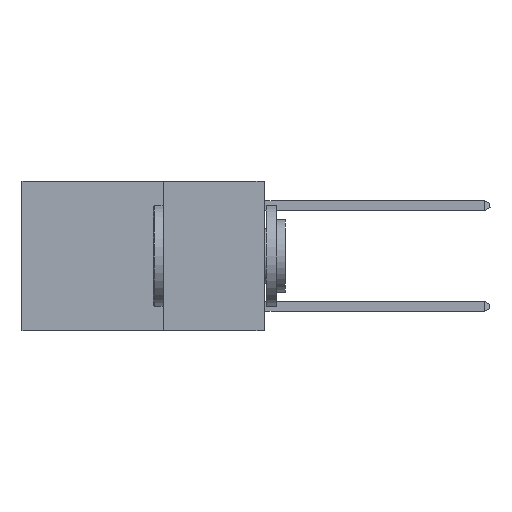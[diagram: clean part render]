
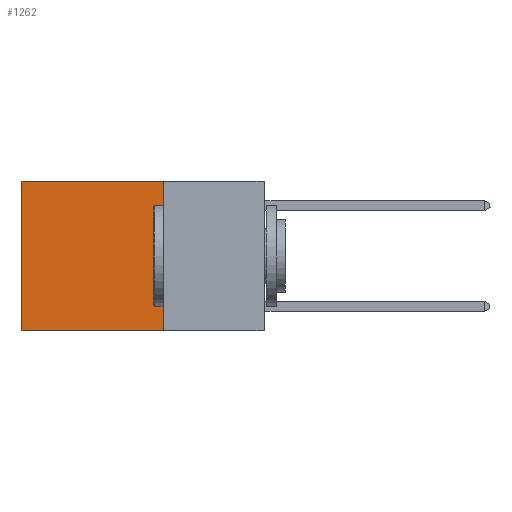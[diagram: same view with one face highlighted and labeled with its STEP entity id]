
A CAD part, left-side view. The second image highlights one B-rep face of the part: STEP entity #1262.
In plain terms, the highlighted planar face has unit normal (-1, 0, 0).
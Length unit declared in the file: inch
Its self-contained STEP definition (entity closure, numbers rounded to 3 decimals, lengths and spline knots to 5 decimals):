
#293 = VECTOR ( 'NONE', #6387, 39.37008 ) ;
#1262 = ADVANCED_FACE ( 'NONE', ( #6623 ), #28082, .F. ) ;
#1396 = DIRECTION ( 'NONE',  ( 0., 0., -1. ) ) ;
#1683 = EDGE_CURVE ( 'NONE', #19348, #7926, #13863, .T. ) ;
#2393 = VERTEX_POINT ( 'NONE', #3580 ) ;
#2856 = DIRECTION ( 'NONE',  ( 0., 1., 0. ) ) ;
#3421 = ORIENTED_EDGE ( 'NONE', *, *, #1683, .T. ) ;
#3580 = CARTESIAN_POINT ( 'NONE',  ( 0.2625, 0.25, 0. ) ) ;
#6175 = LINE ( 'NONE', #24043, #293 ) ;
#6387 = DIRECTION ( 'NONE',  ( 0., 1., 0. ) ) ;
#6623 = FACE_OUTER_BOUND ( 'NONE', #16800, .T. ) ;
#7926 = VERTEX_POINT ( 'NONE', #9619 ) ;
#8200 = ORIENTED_EDGE ( 'NONE', *, *, #11585, .F. ) ;
#8215 = CARTESIAN_POINT ( 'NONE',  ( 0.2625, 0.6, 0. ) ) ;
#9619 = CARTESIAN_POINT ( 'NONE',  ( 0.2625, 0.6, -0.37 ) ) ;
#9666 = LINE ( 'NONE', #28110, #13452 ) ;
#9879 = EDGE_CURVE ( 'NONE', #2393, #19348, #6175, .T. ) ;
#10046 = ORIENTED_EDGE ( 'NONE', *, *, #10754, .F. ) ;
#10754 = EDGE_CURVE ( 'NONE', #14430, #7926, #17958, .T. ) ;
#10755 = VECTOR ( 'NONE', #11783, 39.37008 ) ;
#11585 = EDGE_CURVE ( 'NONE', #2393, #14430, #9666, .T. ) ;
#11783 = DIRECTION ( 'NONE',  ( 0., 0., -1. ) ) ;
#12559 = ORIENTED_EDGE ( 'NONE', *, *, #9879, .T. ) ;
#13452 = VECTOR ( 'NONE', #18923, 39.37008 ) ;
#13863 = LINE ( 'NONE', #19925, #10755 ) ;
#14430 = VERTEX_POINT ( 'NONE', #15342 ) ;
#15342 = CARTESIAN_POINT ( 'NONE',  ( 0.2625, 0.25, -0.37 ) ) ;
#16800 = EDGE_LOOP ( 'NONE', ( #3421, #10046, #8200, #12559 ) ) ;
#17460 = AXIS2_PLACEMENT_3D ( 'NONE', #25722, #23206, #1396 ) ;
#17958 = LINE ( 'NONE', #18425, #19843 ) ;
#18425 = CARTESIAN_POINT ( 'NONE',  ( 0.2625, 0.25, -0.37 ) ) ;
#18923 = DIRECTION ( 'NONE',  ( 0., 0., -1. ) ) ;
#19348 = VERTEX_POINT ( 'NONE', #8215 ) ;
#19843 = VECTOR ( 'NONE', #2856, 39.37008 ) ;
#19925 = CARTESIAN_POINT ( 'NONE',  ( 0.2625, 0.6, 0. ) ) ;
#23206 = DIRECTION ( 'NONE',  ( 1., 0., 0. ) ) ;
#24043 = CARTESIAN_POINT ( 'NONE',  ( 0.2625, 0.25, 0. ) ) ;
#25722 = CARTESIAN_POINT ( 'NONE',  ( 0.2625, 0.25, 0. ) ) ;
#28082 = PLANE ( 'NONE',  #17460 ) ;
#28110 = CARTESIAN_POINT ( 'NONE',  ( 0.2625, 0.25, 0. ) ) ;
